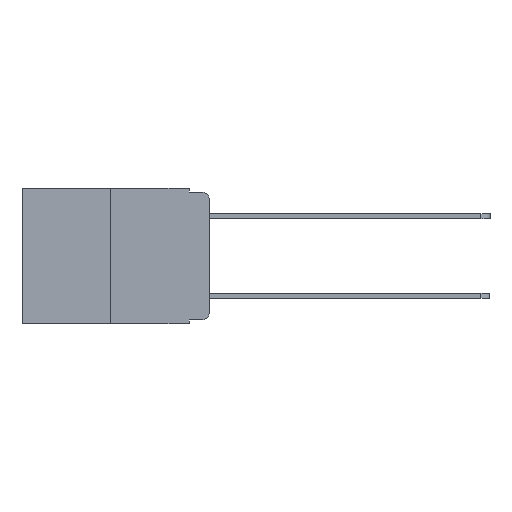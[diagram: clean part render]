
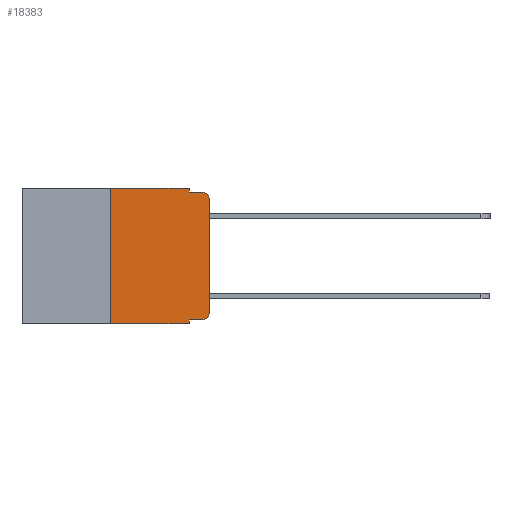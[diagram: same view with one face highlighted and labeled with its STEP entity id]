
A CAD part, left-side view. The second image highlights one B-rep face of the part: STEP entity #18383.
In plain terms, the highlighted planar face has unit normal (-1, 0, 0).
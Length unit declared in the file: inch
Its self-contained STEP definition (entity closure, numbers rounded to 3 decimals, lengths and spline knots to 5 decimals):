
#284 = DIRECTION ( 'NONE',  ( 0., 0., -1. ) ) ;
#889 = VERTEX_POINT ( 'NONE', #15399 ) ;
#1270 = DIRECTION ( 'NONE',  ( 0., -1., 0. ) ) ;
#1390 = ORIENTED_EDGE ( 'NONE', *, *, #21890, .F. ) ;
#1570 = DIRECTION ( 'NONE',  ( 0., -1., 0. ) ) ;
#1620 = LINE ( 'NONE', #13118, #11902 ) ;
#2336 = VERTEX_POINT ( 'NONE', #13046 ) ;
#3159 = CARTESIAN_POINT ( 'NONE',  ( 0., 0.051, -0.343 ) ) ;
#3304 = VECTOR ( 'NONE', #6571, 39.37008 ) ;
#3701 = CARTESIAN_POINT ( 'NONE',  ( 0., 0.051, 0. ) ) ;
#3842 = ORIENTED_EDGE ( 'NONE', *, *, #21863, .T. ) ;
#3877 = VERTEX_POINT ( 'NONE', #6185 ) ;
#4122 = ORIENTED_EDGE ( 'NONE', *, *, #13861, .F. ) ;
#4305 = CARTESIAN_POINT ( 'NONE',  ( 0., 0.051, 0. ) ) ;
#4606 = CARTESIAN_POINT ( 'NONE',  ( 0., 0.051, 0. ) ) ;
#4730 = LINE ( 'NONE', #10776, #18745 ) ;
#4820 = DIRECTION ( 'NONE',  ( 0., -1., 0. ) ) ;
#5351 = ORIENTED_EDGE ( 'NONE', *, *, #15341, .F. ) ;
#5988 = VERTEX_POINT ( 'NONE', #11183 ) ;
#6185 = CARTESIAN_POINT ( 'NONE',  ( 0., 0.051, -0.333 ) ) ;
#6212 = DIRECTION ( 'NONE',  ( 0., 0., 1. ) ) ;
#6264 = DIRECTION ( 'NONE',  ( 0., 0., -1. ) ) ;
#6325 = LINE ( 'NONE', #4305, #14074 ) ;
#6571 = DIRECTION ( 'NONE',  ( 0., 0., -1. ) ) ;
#6579 = DIRECTION ( 'NONE',  ( 0., 0., -1. ) ) ;
#6861 = ORIENTED_EDGE ( 'NONE', *, *, #18818, .T. ) ;
#7631 = VECTOR ( 'NONE', #6212, 39.37008 ) ;
#8006 = LINE ( 'NONE', #14353, #17487 ) ;
#8134 = EDGE_CURVE ( 'NONE', #3877, #12487, #4730, .T. ) ;
#8451 = FACE_OUTER_BOUND ( 'NONE', #23076, .T. ) ;
#8705 = EDGE_CURVE ( 'NONE', #24564, #889, #12520, .T. ) ;
#9422 = CARTESIAN_POINT ( 'NONE',  ( 0., 0., 0. ) ) ;
#9570 = EDGE_CURVE ( 'NONE', #13566, #10354, #8006, .T. ) ;
#9850 = DIRECTION ( 'NONE',  ( -1., 0., 0. ) ) ;
#10354 = VERTEX_POINT ( 'NONE', #3159 ) ;
#10494 = ORIENTED_EDGE ( 'NONE', *, *, #9570, .T. ) ;
#10545 = DIRECTION ( 'NONE',  ( 0., -1., 0. ) ) ;
#10776 = CARTESIAN_POINT ( 'NONE',  ( 0., 0.051, -0.333 ) ) ;
#11183 = CARTESIAN_POINT ( 'NONE',  ( 0., 0.25, 0. ) ) ;
#11719 = EDGE_CURVE ( 'NONE', #24451, #24564, #22893, .T. ) ;
#11902 = VECTOR ( 'NONE', #1570, 39.37008 ) ;
#11905 = DIRECTION ( 'NONE',  ( -1., 0., 0. ) ) ;
#12047 = CIRCLE ( 'NONE', #15538, 0.02 ) ;
#12269 = ORIENTED_EDGE ( 'NONE', *, *, #8134, .T. ) ;
#12346 = CARTESIAN_POINT ( 'NONE',  ( 0., 0.02, -0.333 ) ) ;
#12487 = VERTEX_POINT ( 'NONE', #12346 ) ;
#12520 = LINE ( 'NONE', #18151, #13139 ) ;
#12880 = CIRCLE ( 'NONE', #23923, 0.02 ) ;
#13046 = CARTESIAN_POINT ( 'NONE',  ( 0., 0., -0.313 ) ) ;
#13118 = CARTESIAN_POINT ( 'NONE',  ( 0., 0.473, 0. ) ) ;
#13136 = AXIS2_PLACEMENT_3D ( 'NONE', #21634, #17953, #6579 ) ;
#13139 = VECTOR ( 'NONE', #4820, 39.37008 ) ;
#13459 = CARTESIAN_POINT ( 'NONE',  ( 0., 0., -0.03 ) ) ;
#13466 = VERTEX_POINT ( 'NONE', #13459 ) ;
#13566 = VERTEX_POINT ( 'NONE', #15593 ) ;
#13861 = EDGE_CURVE ( 'NONE', #5988, #24451, #1620, .T. ) ;
#14074 = VECTOR ( 'NONE', #6264, 39.37008 ) ;
#14353 = CARTESIAN_POINT ( 'NONE',  ( 0., 0.473, -0.343 ) ) ;
#14632 = ORIENTED_EDGE ( 'NONE', *, *, #23791, .T. ) ;
#15341 = EDGE_CURVE ( 'NONE', #13566, #5988, #18313, .T. ) ;
#15399 = CARTESIAN_POINT ( 'NONE',  ( 0., 0.02, -0.01 ) ) ;
#15538 = AXIS2_PLACEMENT_3D ( 'NONE', #23104, #11905, #284 ) ;
#15593 = CARTESIAN_POINT ( 'NONE',  ( 0., 0.25, -0.343 ) ) ;
#16062 = PLANE ( 'NONE',  #13136 ) ;
#16952 = ORIENTED_EDGE ( 'NONE', *, *, #8705, .F. ) ;
#17487 = VECTOR ( 'NONE', #10545, 39.37008 ) ;
#17953 = DIRECTION ( 'NONE',  ( 1., 0., 0. ) ) ;
#18151 = CARTESIAN_POINT ( 'NONE',  ( 0., 0.051, -0.01 ) ) ;
#18153 = ORIENTED_EDGE ( 'NONE', *, *, #11719, .F. ) ;
#18313 = LINE ( 'NONE', #23135, #7631 ) ;
#18383 = ADVANCED_FACE ( 'NONE', ( #8451 ), #16062, .F. ) ;
#18745 = VECTOR ( 'NONE', #1270, 39.37008 ) ;
#18818 = EDGE_CURVE ( 'NONE', #13466, #889, #12880, .T. ) ;
#19233 = VECTOR ( 'NONE', #22568, 39.37008 ) ;
#21123 = CARTESIAN_POINT ( 'NONE',  ( 0., 0.02, -0.03 ) ) ;
#21634 = CARTESIAN_POINT ( 'NONE',  ( 0., 0.473, 0. ) ) ;
#21863 = EDGE_CURVE ( 'NONE', #12487, #2336, #12047, .T. ) ;
#21890 = EDGE_CURVE ( 'NONE', #3877, #10354, #6325, .T. ) ;
#22568 = DIRECTION ( 'NONE',  ( 0., 0., 1. ) ) ;
#22893 = LINE ( 'NONE', #4606, #3304 ) ;
#22997 = DIRECTION ( 'NONE',  ( 0., 0., -1. ) ) ;
#23011 = CARTESIAN_POINT ( 'NONE',  ( 0., 0.051, -0.01 ) ) ;
#23076 = EDGE_LOOP ( 'NONE', ( #14632, #6861, #16952, #18153, #4122, #5351, #10494, #1390, #12269, #3842 ) ) ;
#23104 = CARTESIAN_POINT ( 'NONE',  ( 0., 0.02, -0.313 ) ) ;
#23135 = CARTESIAN_POINT ( 'NONE',  ( 0., 0.25, 0. ) ) ;
#23791 = EDGE_CURVE ( 'NONE', #2336, #13466, #24174, .T. ) ;
#23923 = AXIS2_PLACEMENT_3D ( 'NONE', #21123, #9850, #22997 ) ;
#24174 = LINE ( 'NONE', #9422, #19233 ) ;
#24451 = VERTEX_POINT ( 'NONE', #3701 ) ;
#24564 = VERTEX_POINT ( 'NONE', #23011 ) ;
